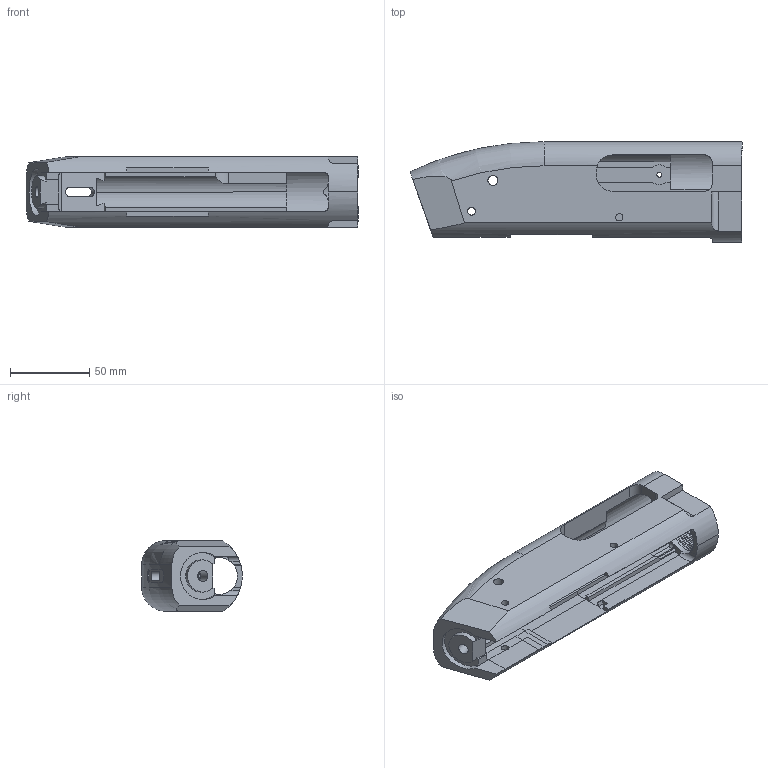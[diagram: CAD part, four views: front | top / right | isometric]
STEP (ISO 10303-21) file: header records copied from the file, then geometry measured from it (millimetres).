
FILE_DESCRIPTION(('FreeCAD Model'),'2;1');
FILE_NAME('Open CASCADE Shape Model','2023-01-12T22:10:32',('Author'),( ''),'Open CASCADE STEP processor 7.5','FreeCAD','Unknown');
FILE_SCHEMA(('AUTOMOTIVE_DESIGN { 1 0 10303 214 1 1 1 1 }'));
Length unit declared in the file: millimetre
Products named in the file (1): Pocket028
Bounding box: 209.55 x 63.5 x 44.45 mm (x, y, z)
Volume: 201929.7 mm3; surface area: 64931.2 mm2
Topology: 1 solids, 1 shells, 233 faces, 665 edges, 427 vertices
Faces by surface type: plane 154, cylinder 56, bspline 21, torus 2
Full cylindrical faces by diameter (mm): 3.048 x1, 4.572 x1, 4.826 x2, 6.35 x2, 6.858 x1, 23.114 x1, 24.384 x6, 32.766 x1
Entity records: 23976 total; most frequent: CARTESIAN_POINT 11699, DIRECTION 1973, ORIENTED_EDGE 1330, PCURVE 1330, DEFINITIONAL_REPRESENTATION 1330, LINE 1173, VECTOR 1173, EDGE_CURVE 665
